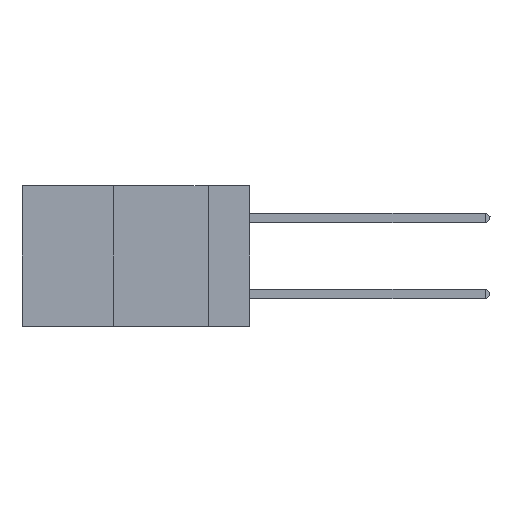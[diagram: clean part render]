
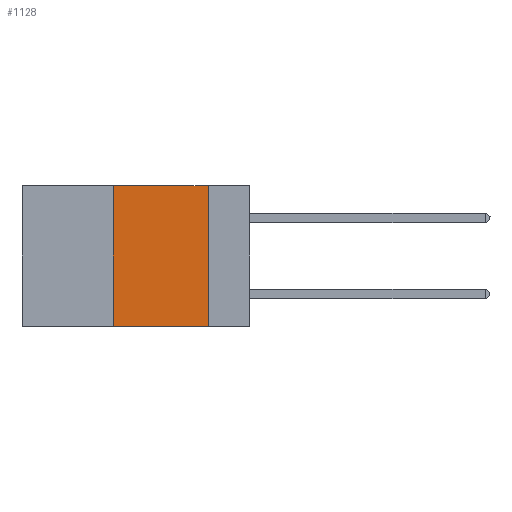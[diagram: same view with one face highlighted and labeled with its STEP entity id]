
A CAD part, left-side view. The second image highlights one B-rep face of the part: STEP entity #1128.
In plain terms, the highlighted planar face has unit normal (-1, 0, 0).
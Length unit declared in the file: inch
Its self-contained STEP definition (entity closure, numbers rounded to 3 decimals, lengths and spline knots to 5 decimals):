
#64 = EDGE_CURVE ( 'NONE', #3505, #150, #3369, .T. ) ;
#150 = VERTEX_POINT ( 'NONE', #6766 ) ;
#207 = CARTESIAN_POINT ( 'NONE',  ( 0., 0.11, 0. ) ) ;
#389 = ORIENTED_EDGE ( 'NONE', *, *, #64, .T. ) ;
#673 = CARTESIAN_POINT ( 'NONE',  ( 0., 0.11, 0. ) ) ;
#1118 = ORIENTED_EDGE ( 'NONE', *, *, #8060, .F. ) ;
#1128 = ADVANCED_FACE ( 'NONE', ( #8960 ), #6067, .F. ) ;
#1654 = EDGE_CURVE ( 'NONE', #3505, #3363, #8463, .T. ) ;
#1977 = CARTESIAN_POINT ( 'NONE',  ( 0., 0.36, 0. ) ) ;
#1997 = VERTEX_POINT ( 'NONE', #207 ) ;
#3363 = VERTEX_POINT ( 'NONE', #6096 ) ;
#3369 = LINE ( 'NONE', #8266, #5695 ) ;
#3505 = VERTEX_POINT ( 'NONE', #6649 ) ;
#3693 = EDGE_LOOP ( 'NONE', ( #8379, #1118, #6279, #389 ) ) ;
#3778 = DIRECTION ( 'NONE',  ( 0., -1., 0. ) ) ;
#4330 = LINE ( 'NONE', #7730, #9475 ) ;
#5451 = LINE ( 'NONE', #673, #7203 ) ;
#5695 = VECTOR ( 'NONE', #3778, 39.37008 ) ;
#6067 = PLANE ( 'NONE',  #9197 ) ;
#6096 = CARTESIAN_POINT ( 'NONE',  ( 0., 0.36, 0. ) ) ;
#6279 = ORIENTED_EDGE ( 'NONE', *, *, #1654, .F. ) ;
#6354 = CARTESIAN_POINT ( 'NONE',  ( 0., 0.6, 0. ) ) ;
#6489 = VECTOR ( 'NONE', #7978, 39.37008 ) ;
#6649 = CARTESIAN_POINT ( 'NONE',  ( 0., 0.36, -0.37 ) ) ;
#6688 = DIRECTION ( 'NONE',  ( 0., 0., -1. ) ) ;
#6766 = CARTESIAN_POINT ( 'NONE',  ( 0., 0.11, -0.37 ) ) ;
#7203 = VECTOR ( 'NONE', #8269, 39.37008 ) ;
#7730 = CARTESIAN_POINT ( 'NONE',  ( 0., 0.6, 0. ) ) ;
#7978 = DIRECTION ( 'NONE',  ( 0., 0., 1. ) ) ;
#8060 = EDGE_CURVE ( 'NONE', #3363, #1997, #4330, .T. ) ;
#8266 = CARTESIAN_POINT ( 'NONE',  ( 0., 0.6, -0.37 ) ) ;
#8269 = DIRECTION ( 'NONE',  ( 0., 0., -1. ) ) ;
#8352 = EDGE_CURVE ( 'NONE', #1997, #150, #5451, .T. ) ;
#8379 = ORIENTED_EDGE ( 'NONE', *, *, #8352, .F. ) ;
#8463 = LINE ( 'NONE', #1977, #6489 ) ;
#8960 = FACE_OUTER_BOUND ( 'NONE', #3693, .T. ) ;
#9197 = AXIS2_PLACEMENT_3D ( 'NONE', #6354, #9634, #6688 ) ;
#9219 = DIRECTION ( 'NONE',  ( 0., -1., 0. ) ) ;
#9475 = VECTOR ( 'NONE', #9219, 39.37008 ) ;
#9634 = DIRECTION ( 'NONE',  ( 1., 0., 0. ) ) ;
